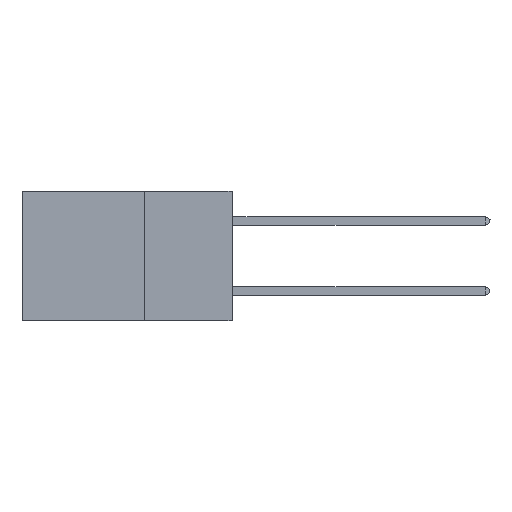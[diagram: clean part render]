
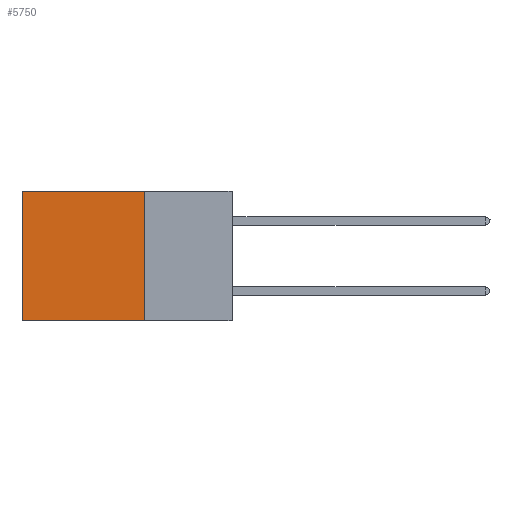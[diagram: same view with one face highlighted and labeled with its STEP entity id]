
A CAD part, left-side view. The second image highlights one B-rep face of the part: STEP entity #5750.
In plain terms, the highlighted planar face has unit normal (-1, 0, 0).
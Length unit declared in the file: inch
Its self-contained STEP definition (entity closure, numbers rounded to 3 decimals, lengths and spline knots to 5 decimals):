
#159 = VERTEX_POINT ( 'NONE', #1458 ) ;
#269 = LINE ( 'NONE', #15619, #14797 ) ;
#343 = DIRECTION ( 'NONE',  ( 1., 0., 0. ) ) ;
#1321 = CARTESIAN_POINT ( 'NONE',  ( 0.2875, 0.6, 0. ) ) ;
#1458 = CARTESIAN_POINT ( 'NONE',  ( 0.2875, 0.25, 0. ) ) ;
#1741 = EDGE_CURVE ( 'NONE', #159, #15063, #269, .T. ) ;
#1754 = CARTESIAN_POINT ( 'NONE',  ( 0.2875, 0.6, -0.37 ) ) ;
#1914 = VERTEX_POINT ( 'NONE', #1754 ) ;
#1919 = DIRECTION ( 'NONE',  ( 0., 1., 0. ) ) ;
#3312 = VECTOR ( 'NONE', #10764, 39.37008 ) ;
#4526 = EDGE_CURVE ( 'NONE', #159, #16237, #17688, .T. ) ;
#5030 = CARTESIAN_POINT ( 'NONE',  ( 0.2875, 0.25, 0. ) ) ;
#5559 = LINE ( 'NONE', #1321, #12173 ) ;
#5750 = ADVANCED_FACE ( 'NONE', ( #13108 ), #7365, .F. ) ;
#5908 = DIRECTION ( 'NONE',  ( 0., 0., -1. ) ) ;
#7365 = PLANE ( 'NONE',  #18106 ) ;
#7652 = LINE ( 'NONE', #9127, #9675 ) ;
#8110 = ORIENTED_EDGE ( 'NONE', *, *, #12751, .F. ) ;
#8514 = ORIENTED_EDGE ( 'NONE', *, *, #4526, .T. ) ;
#9127 = CARTESIAN_POINT ( 'NONE',  ( 0.2875, 0.25, -0.37 ) ) ;
#9675 = VECTOR ( 'NONE', #1919, 39.37008 ) ;
#10764 = DIRECTION ( 'NONE',  ( 0., 1., 0. ) ) ;
#11579 = CARTESIAN_POINT ( 'NONE',  ( 0.2875, 0.25, -0.37 ) ) ;
#11621 = CARTESIAN_POINT ( 'NONE',  ( 0.2875, 0.25, 0. ) ) ;
#12173 = VECTOR ( 'NONE', #12677, 39.37008 ) ;
#12659 = EDGE_LOOP ( 'NONE', ( #15366, #8110, #15251, #8514 ) ) ;
#12677 = DIRECTION ( 'NONE',  ( 0., 0., -1. ) ) ;
#12751 = EDGE_CURVE ( 'NONE', #15063, #1914, #7652, .T. ) ;
#13108 = FACE_OUTER_BOUND ( 'NONE', #12659, .T. ) ;
#14797 = VECTOR ( 'NONE', #5908, 39.37008 ) ;
#15063 = VERTEX_POINT ( 'NONE', #11579 ) ;
#15251 = ORIENTED_EDGE ( 'NONE', *, *, #1741, .F. ) ;
#15335 = EDGE_CURVE ( 'NONE', #16237, #1914, #5559, .T. ) ;
#15366 = ORIENTED_EDGE ( 'NONE', *, *, #15335, .T. ) ;
#15619 = CARTESIAN_POINT ( 'NONE',  ( 0.2875, 0.25, 0. ) ) ;
#16237 = VERTEX_POINT ( 'NONE', #16948 ) ;
#16948 = CARTESIAN_POINT ( 'NONE',  ( 0.2875, 0.6, 0. ) ) ;
#17251 = DIRECTION ( 'NONE',  ( 0., 0., -1. ) ) ;
#17688 = LINE ( 'NONE', #5030, #3312 ) ;
#18106 = AXIS2_PLACEMENT_3D ( 'NONE', #11621, #343, #17251 ) ;
